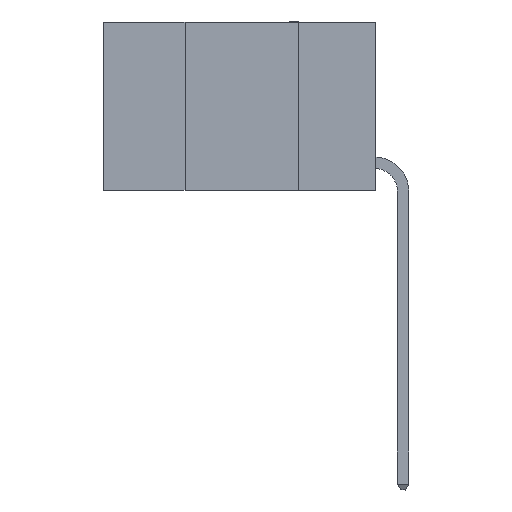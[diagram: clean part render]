
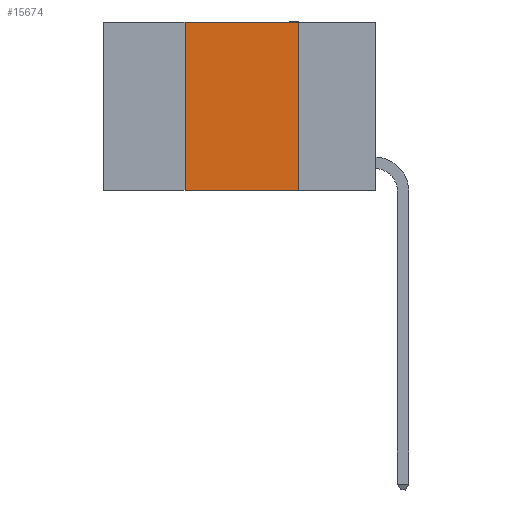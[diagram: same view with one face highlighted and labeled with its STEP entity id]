
A CAD part, left-side view. The second image highlights one B-rep face of the part: STEP entity #15674.
In plain terms, the highlighted planar face has unit normal (-1, 0, 0).
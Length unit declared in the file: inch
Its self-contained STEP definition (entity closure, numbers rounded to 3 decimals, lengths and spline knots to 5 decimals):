
#662 = FACE_OUTER_BOUND ( 'NONE', #9142, .T. ) ;
#2065 = VECTOR ( 'NONE', #10474, 39.37008 ) ;
#2501 = CARTESIAN_POINT ( 'NONE',  ( 0., 0.17, 0. ) ) ;
#2712 = VERTEX_POINT ( 'NONE', #14992 ) ;
#2792 = CARTESIAN_POINT ( 'NONE',  ( 0., 0.6, -0.37 ) ) ;
#3076 = LINE ( 'NONE', #2792, #20408 ) ;
#3109 = CARTESIAN_POINT ( 'NONE',  ( 0., 0.17, -0.37 ) ) ;
#4717 = VECTOR ( 'NONE', #9985, 39.37008 ) ;
#7351 = DIRECTION ( 'NONE',  ( 1., 0., 0. ) ) ;
#8141 = CARTESIAN_POINT ( 'NONE',  ( 0., 0.6, 0. ) ) ;
#8189 = DIRECTION ( 'NONE',  ( 0., -1., 0. ) ) ;
#9142 = EDGE_LOOP ( 'NONE', ( #11774, #16522, #21202, #12333 ) ) ;
#9985 = DIRECTION ( 'NONE',  ( 0., -1., 0. ) ) ;
#10413 = CARTESIAN_POINT ( 'NONE',  ( 0., 0.42, 0. ) ) ;
#10474 = DIRECTION ( 'NONE',  ( 0., 0., 1. ) ) ;
#10809 = CARTESIAN_POINT ( 'NONE',  ( 0., 0.6, 0. ) ) ;
#11086 = LINE ( 'NONE', #19329, #2065 ) ;
#11774 = ORIENTED_EDGE ( 'NONE', *, *, #17041, .F. ) ;
#11965 = VERTEX_POINT ( 'NONE', #12888 ) ;
#12333 = ORIENTED_EDGE ( 'NONE', *, *, #18217, .T. ) ;
#12888 = CARTESIAN_POINT ( 'NONE',  ( 0., 0.17, 0. ) ) ;
#13055 = VERTEX_POINT ( 'NONE', #10413 ) ;
#14096 = EDGE_CURVE ( 'NONE', #13055, #11965, #18975, .T. ) ;
#14685 = LINE ( 'NONE', #2501, #22938 ) ;
#14992 = CARTESIAN_POINT ( 'NONE',  ( 0., 0.42, -0.37 ) ) ;
#15674 = ADVANCED_FACE ( 'NONE', ( #662 ), #18027, .F. ) ;
#16056 = EDGE_CURVE ( 'NONE', #2712, #13055, #11086, .T. ) ;
#16522 = ORIENTED_EDGE ( 'NONE', *, *, #14096, .F. ) ;
#17041 = EDGE_CURVE ( 'NONE', #11965, #19598, #14685, .T. ) ;
#17977 = AXIS2_PLACEMENT_3D ( 'NONE', #10809, #7351, #19799 ) ;
#18027 = PLANE ( 'NONE',  #17977 ) ;
#18217 = EDGE_CURVE ( 'NONE', #2712, #19598, #3076, .T. ) ;
#18975 = LINE ( 'NONE', #8141, #4717 ) ;
#19329 = CARTESIAN_POINT ( 'NONE',  ( 0., 0.42, 0. ) ) ;
#19598 = VERTEX_POINT ( 'NONE', #3109 ) ;
#19799 = DIRECTION ( 'NONE',  ( 0., 0., -1. ) ) ;
#20408 = VECTOR ( 'NONE', #8189, 39.37008 ) ;
#21202 = ORIENTED_EDGE ( 'NONE', *, *, #16056, .F. ) ;
#22068 = DIRECTION ( 'NONE',  ( 0., 0., -1. ) ) ;
#22938 = VECTOR ( 'NONE', #22068, 39.37008 ) ;
